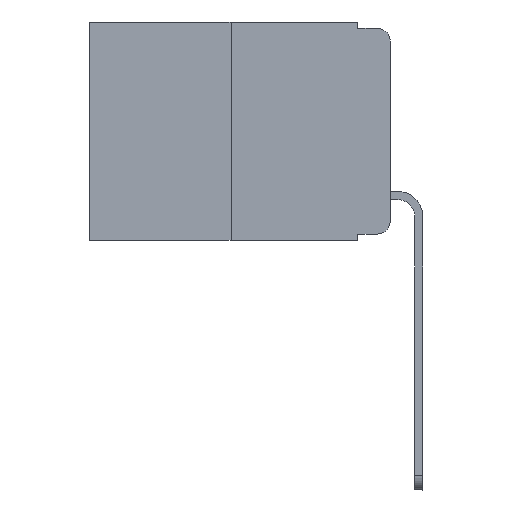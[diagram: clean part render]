
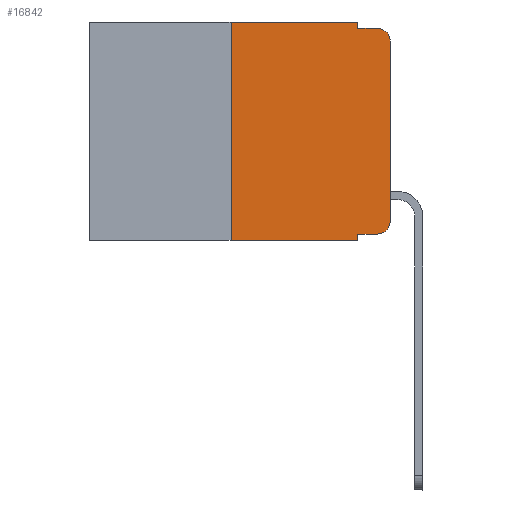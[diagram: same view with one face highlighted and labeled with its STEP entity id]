
A CAD part, left-side view. The second image highlights one B-rep face of the part: STEP entity #16842.
In plain terms, the highlighted planar face has unit normal (-1, 0, 0).
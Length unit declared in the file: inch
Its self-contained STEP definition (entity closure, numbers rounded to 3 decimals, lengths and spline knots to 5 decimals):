
#207 = ORIENTED_EDGE ( 'NONE', *, *, #19982, .F. ) ;
#423 = ORIENTED_EDGE ( 'NONE', *, *, #13400, .F. ) ;
#431 = CARTESIAN_POINT ( 'NONE',  ( 0., 0.051, 0. ) ) ;
#550 = DIRECTION ( 'NONE',  ( 0., 0., -1. ) ) ;
#589 = ORIENTED_EDGE ( 'NONE', *, *, #12583, .F. ) ;
#730 = CARTESIAN_POINT ( 'NONE',  ( 0., 0.051, -0.333 ) ) ;
#1065 = CARTESIAN_POINT ( 'NONE',  ( 0., 0.02, -0.01 ) ) ;
#1827 = DIRECTION ( 'NONE',  ( 0., 0., 1. ) ) ;
#1988 = VECTOR ( 'NONE', #6263, 39.37008 ) ;
#2220 = CARTESIAN_POINT ( 'NONE',  ( 0., 0.051, -0.01 ) ) ;
#3267 = VERTEX_POINT ( 'NONE', #1065 ) ;
#3390 = DIRECTION ( 'NONE',  ( 0., 0., -1. ) ) ;
#3445 = CARTESIAN_POINT ( 'NONE',  ( 0., 0.02, -0.333 ) ) ;
#3775 = LINE ( 'NONE', #21319, #6402 ) ;
#3882 = VECTOR ( 'NONE', #6513, 39.37008 ) ;
#4019 = ORIENTED_EDGE ( 'NONE', *, *, #15181, .T. ) ;
#4089 = DIRECTION ( 'NONE',  ( -1., 0., 0. ) ) ;
#4405 = ORIENTED_EDGE ( 'NONE', *, *, #21529, .T. ) ;
#4499 = CIRCLE ( 'NONE', #20250, 0.02 ) ;
#5545 = CARTESIAN_POINT ( 'NONE',  ( 0., 0.051, 0. ) ) ;
#5563 = CARTESIAN_POINT ( 'NONE',  ( 0., 0.02, -0.313 ) ) ;
#5779 = EDGE_CURVE ( 'NONE', #22068, #3267, #20121, .T. ) ;
#5968 = EDGE_CURVE ( 'NONE', #9776, #8432, #7322, .T. ) ;
#6263 = DIRECTION ( 'NONE',  ( 0., 0., 1. ) ) ;
#6402 = VECTOR ( 'NONE', #10757, 39.37008 ) ;
#6490 = CARTESIAN_POINT ( 'NONE',  ( 0., 0.25, 0. ) ) ;
#6513 = DIRECTION ( 'NONE',  ( 0., 0., -1. ) ) ;
#7322 = LINE ( 'NONE', #17542, #9912 ) ;
#7574 = DIRECTION ( 'NONE',  ( 0., -1., 0. ) ) ;
#8177 = CARTESIAN_POINT ( 'NONE',  ( 0., 0.051, -0.01 ) ) ;
#8432 = VERTEX_POINT ( 'NONE', #22532 ) ;
#9058 = LINE ( 'NONE', #730, #11378 ) ;
#9102 = DIRECTION ( 'NONE',  ( -1., 0., 0. ) ) ;
#9338 = EDGE_CURVE ( 'NONE', #13579, #19250, #12241, .T. ) ;
#9544 = VECTOR ( 'NONE', #18615, 39.37008 ) ;
#9636 = ORIENTED_EDGE ( 'NONE', *, *, #19346, .F. ) ;
#9776 = VERTEX_POINT ( 'NONE', #10809 ) ;
#9780 = VECTOR ( 'NONE', #1827, 39.37008 ) ;
#9912 = VECTOR ( 'NONE', #19367, 39.37008 ) ;
#10135 = CARTESIAN_POINT ( 'NONE',  ( 0., 0.25, 0. ) ) ;
#10757 = DIRECTION ( 'NONE',  ( 0., -1., 0. ) ) ;
#10798 = CIRCLE ( 'NONE', #18893, 0.02 ) ;
#10809 = CARTESIAN_POINT ( 'NONE',  ( 0., 0.25, -0.343 ) ) ;
#11378 = VECTOR ( 'NONE', #7574, 39.37008 ) ;
#12241 = LINE ( 'NONE', #15955, #9780 ) ;
#12451 = VECTOR ( 'NONE', #550, 39.37008 ) ;
#12583 = EDGE_CURVE ( 'NONE', #17070, #8432, #22229, .T. ) ;
#12593 = CARTESIAN_POINT ( 'NONE',  ( 0., 0.473, 0. ) ) ;
#12913 = DIRECTION ( 'NONE',  ( 0., 0., -1. ) ) ;
#13400 = EDGE_CURVE ( 'NONE', #13401, #22068, #16241, .T. ) ;
#13401 = VERTEX_POINT ( 'NONE', #431 ) ;
#13463 = EDGE_LOOP ( 'NONE', ( #19537, #4405, #13781, #423, #9636, #207, #15377, #589, #4019, #20713 ) ) ;
#13579 = VERTEX_POINT ( 'NONE', #21728 ) ;
#13748 = CARTESIAN_POINT ( 'NONE',  ( 0., 0.051, -0.333 ) ) ;
#13781 = ORIENTED_EDGE ( 'NONE', *, *, #5779, .F. ) ;
#14463 = CARTESIAN_POINT ( 'NONE',  ( 0., 0., -0.03 ) ) ;
#15131 = AXIS2_PLACEMENT_3D ( 'NONE', #12593, #21662, #19598 ) ;
#15181 = EDGE_CURVE ( 'NONE', #17070, #19074, #9058, .T. ) ;
#15377 = ORIENTED_EDGE ( 'NONE', *, *, #5968, .T. ) ;
#15955 = CARTESIAN_POINT ( 'NONE',  ( 0., 0., 0. ) ) ;
#16241 = LINE ( 'NONE', #5545, #12451 ) ;
#16842 = ADVANCED_FACE ( 'NONE', ( #21553 ), #21431, .F. ) ;
#17070 = VERTEX_POINT ( 'NONE', #13748 ) ;
#17274 = EDGE_CURVE ( 'NONE', #19074, #13579, #4499, .T. ) ;
#17542 = CARTESIAN_POINT ( 'NONE',  ( 0., 0.473, -0.343 ) ) ;
#18615 = DIRECTION ( 'NONE',  ( 0., -1., 0. ) ) ;
#18893 = AXIS2_PLACEMENT_3D ( 'NONE', #19206, #9102, #3390 ) ;
#18978 = LINE ( 'NONE', #10135, #1988 ) ;
#19074 = VERTEX_POINT ( 'NONE', #3445 ) ;
#19206 = CARTESIAN_POINT ( 'NONE',  ( 0., 0.02, -0.03 ) ) ;
#19250 = VERTEX_POINT ( 'NONE', #14463 ) ;
#19346 = EDGE_CURVE ( 'NONE', #20096, #13401, #3775, .T. ) ;
#19367 = DIRECTION ( 'NONE',  ( 0., -1., 0. ) ) ;
#19537 = ORIENTED_EDGE ( 'NONE', *, *, #9338, .T. ) ;
#19598 = DIRECTION ( 'NONE',  ( 0., 0., -1. ) ) ;
#19982 = EDGE_CURVE ( 'NONE', #9776, #20096, #18978, .T. ) ;
#20096 = VERTEX_POINT ( 'NONE', #6490 ) ;
#20121 = LINE ( 'NONE', #8177, #9544 ) ;
#20250 = AXIS2_PLACEMENT_3D ( 'NONE', #5563, #4089, #12913 ) ;
#20713 = ORIENTED_EDGE ( 'NONE', *, *, #17274, .T. ) ;
#21319 = CARTESIAN_POINT ( 'NONE',  ( 0., 0.473, 0. ) ) ;
#21431 = PLANE ( 'NONE',  #15131 ) ;
#21529 = EDGE_CURVE ( 'NONE', #19250, #3267, #10798, .T. ) ;
#21553 = FACE_OUTER_BOUND ( 'NONE', #13463, .T. ) ;
#21662 = DIRECTION ( 'NONE',  ( 1., 0., 0. ) ) ;
#21728 = CARTESIAN_POINT ( 'NONE',  ( 0., 0., -0.313 ) ) ;
#22010 = CARTESIAN_POINT ( 'NONE',  ( 0., 0.051, 0. ) ) ;
#22068 = VERTEX_POINT ( 'NONE', #2220 ) ;
#22229 = LINE ( 'NONE', #22010, #3882 ) ;
#22532 = CARTESIAN_POINT ( 'NONE',  ( 0., 0.051, -0.343 ) ) ;
